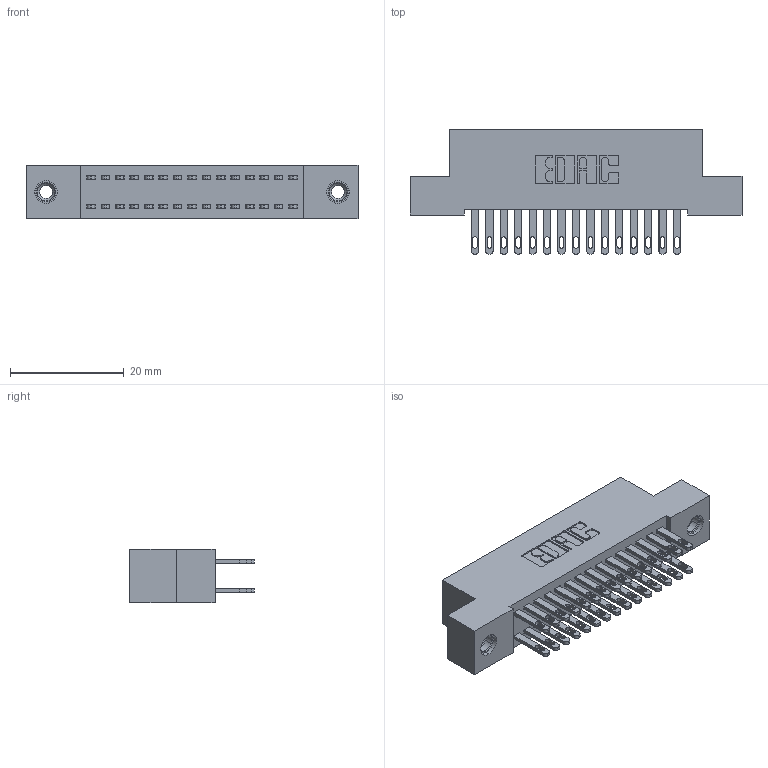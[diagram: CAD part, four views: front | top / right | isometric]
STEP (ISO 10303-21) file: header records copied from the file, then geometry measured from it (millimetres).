
FILE_DESCRIPTION (( 'STEP AP203' ), '1' );
FILE_NAME ('892-030-500-208.STEP', '2020-09-21T15:12:12', ( '' ), ( '' ), 'SwSTEP 2.0', 'SolidWorks 2020', '' );
FILE_SCHEMA (( 'CONFIG_CONTROL_DESIGN' ));
Length unit declared in the file: inch
Products named in the file (4): 892-030-500-208; 345-292-001_345-293-100; 842 Part_TI; 345-250-001_345-250-003-102
Assembly tree (33 placements, depth 2):
  892-030-500-208
    842 Part_TI
    345-292-001_345-293-100  x30
    345-250-001_345-250-003-102  x2
Bounding box: 58.42 x 21.85 x 9.4 mm (x, y, z)
Volume: 5207.2 mm3; surface area: 8108.3 mm2
Topology: 33 solids, 33 shells, 1610 faces, 4845 edges, 3222 vertices
Faces by surface type: plane 998, cylinder 596, cone 12, torus 4
Entity records: 14126 total; most frequent: CARTESIAN_POINT 2353, ORIENTED_EDGE 2282, DIRECTION 2091, EDGE_CURVE 1141, LINE 989, VECTOR 989, VERTEX_POINT 756, AXIS2_PLACEMENT_3D 551
